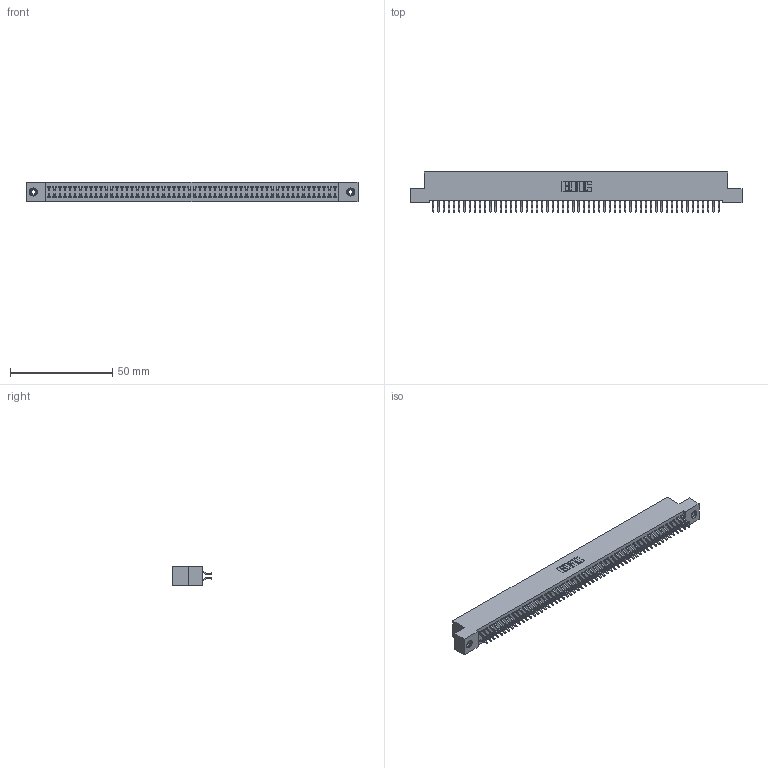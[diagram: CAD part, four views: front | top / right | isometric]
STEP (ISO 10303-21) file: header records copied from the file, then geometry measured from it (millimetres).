
FILE_DESCRIPTION (( 'STEP AP203' ), '1' );
FILE_NAME ('392-112-556-208.STEP', '2018-08-18T22:46:57', ( '' ), ( '' ), 'SwSTEP 2.0', 'SolidWorks 2016', '' );
FILE_SCHEMA (( 'CONFIG_CONTROL_DESIGN' ));
Length unit declared in the file: inch
Products named in the file (4): 345-292-001_556 Tail; 345-250-001_345-250-003-102; 392-112-556-208; 342 Part_TI
Assembly tree (115 placements, depth 2):
  392-112-556-208
    342 Part_TI
    345-292-001_556 Tail  x112
    345-250-001_345-250-003-102  x2
Bounding box: 162.56 x 19.58 x 9.4 mm (x, y, z)
Volume: 14663.7 mm3; surface area: 24115.5 mm2
Topology: 115 solids, 115 shells, 6666 faces, 19811 edges, 13050 vertices
Faces by surface type: plane 4578, cylinder 2072, cone 12, torus 4
Entity records: 35490 total; most frequent: CARTESIAN_POINT 5861, ORIENTED_EDGE 5778, DIRECTION 5003, EDGE_CURVE 2889, VECTOR 2733, LINE 2733, VERTEX_POINT 1920, AXIS2_PLACEMENT_3D 1135
